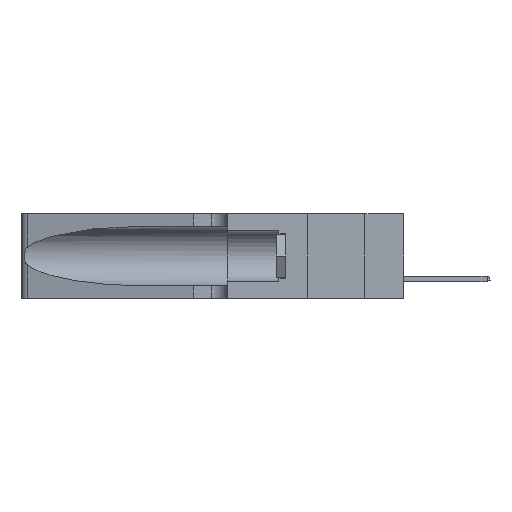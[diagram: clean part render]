
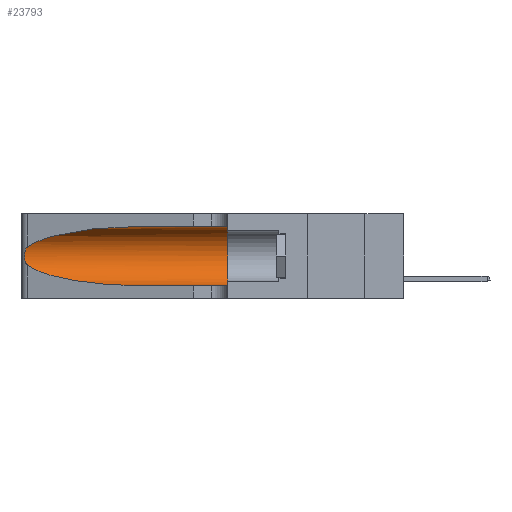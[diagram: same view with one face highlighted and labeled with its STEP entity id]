
A CAD part, left-side view. The second image highlights one B-rep face of the part: STEP entity #23793.
In plain terms, the highlighted cylindrical face has radius 3.308 mm (diameter 6.617 mm), a partial arc.
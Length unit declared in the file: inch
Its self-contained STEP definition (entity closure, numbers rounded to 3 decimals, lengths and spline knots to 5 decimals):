
#1531 = DIRECTION ( 'NONE',  ( 0., -1., 0. ) ) ;
#1923 = CARTESIAN_POINT ( 'NONE',  ( 0.26075, 1.23896, 0.19203 ) ) ;
#2465 = CARTESIAN_POINT ( 'NONE',  ( 0.2373, 1.15595, 0.28018 ) ) ;
#3826 = CARTESIAN_POINT ( 'NONE',  ( 0.1305, 1.61858, 0.31525 ) ) ;
#4246 = LINE ( 'NONE', #3826, #32758 ) ;
#4574 =( BOUNDED_CURVE ( )  B_SPLINE_CURVE ( 3, ( #13751, #26073, #12186, #14116 ),
 .UNSPECIFIED., .F., .F. ) 
 B_SPLINE_CURVE_WITH_KNOTS ( ( 4, 4 ),
 ( 3.44316, 4.71239 ),
 .UNSPECIFIED. ) 
 CURVE ( )  GEOMETRIC_REPRESENTATION_ITEM ( )  RATIONAL_B_SPLINE_CURVE ( ( 1., 0.87, 0.87, 1. ) ) 
 REPRESENTATION_ITEM ( '' )  );
#6546 = CARTESIAN_POINT ( 'NONE',  ( 0.25487, 1.22718, 0.22369 ) ) ;
#7727 = CARTESIAN_POINT ( 'NONE',  ( 0.25787, 1.23484, 0.2124 ) ) ;
#7831 = CARTESIAN_POINT ( 'NONE',  ( 0.25639, 1.23184, 0.21858 ) ) ;
#8335 = ORIENTED_EDGE ( 'NONE', *, *, #14795, .F. ) ;
#8424 = ORIENTED_EDGE ( 'NONE', *, *, #20036, .T. ) ;
#9302 = VERTEX_POINT ( 'NONE', #25267 ) ;
#9339 = CARTESIAN_POINT ( 'NONE',  ( 0.1305, 0.72297, 0.05475 ) ) ;
#10026 = CARTESIAN_POINT ( 'NONE',  ( 0.25487, 1.22718, 0.14631 ) ) ;
#10358 = CARTESIAN_POINT ( 'NONE',  ( 0.25856, 1.23593, 0.16098 ) ) ;
#10730 = CARTESIAN_POINT ( 'NONE',  ( 0.26018, 1.23835, 0.19895 ) ) ;
#10755 = DIRECTION ( 'NONE',  ( 0., 0., -1. ) ) ;
#12186 = CARTESIAN_POINT ( 'NONE',  ( 0.18966, 0.96281, 0.05475 ) ) ;
#12914 = AXIS2_PLACEMENT_3D ( 'NONE', #31276, #17505, #10755 ) ;
#12958 = DIRECTION ( 'NONE',  ( 0., -1., 0. ) ) ;
#12993 = ORIENTED_EDGE ( 'NONE', *, *, #33071, .T. ) ;
#13019 = AXIS2_PLACEMENT_3D ( 'NONE', #30638, #27631, #33396 ) ;
#13751 = CARTESIAN_POINT ( 'NONE',  ( 0.25487, 1.22718, 0.14631 ) ) ;
#13845 = B_SPLINE_CURVE_WITH_KNOTS ( 'NONE', 3,
 ( #24495, #27033, #7831, #7727, #15796, #10730, #1923, #35214, #32194, #10358, #16034, #32328, #32706, #24113 ),
 .UNSPECIFIED., .F., .F.,
 ( 4, 2, 2, 2, 2, 2, 4 ),
 ( 0., 0.00027, 0.00053, 0.00107, 0.0016, 0.00187, 0.00214 ),
 .UNSPECIFIED. ) ;
#14116 = CARTESIAN_POINT ( 'NONE',  ( 0.1305, 0.72297, 0.05475 ) ) ;
#14390 = ORIENTED_EDGE ( 'NONE', *, *, #17416, .F. ) ;
#14795 = EDGE_CURVE ( 'NONE', #35365, #9302, #4246, .T. ) ;
#15796 = CARTESIAN_POINT ( 'NONE',  ( 0.25854, 1.2359, 0.20912 ) ) ;
#16034 = CARTESIAN_POINT ( 'NONE',  ( 0.25789, 1.23486, 0.15765 ) ) ;
#16578 = VERTEX_POINT ( 'NONE', #22984 ) ;
#17416 = EDGE_CURVE ( 'NONE', #9302, #16578, #18355, .T. ) ;
#17505 = DIRECTION ( 'NONE',  ( 0., -1., 0. ) ) ;
#18355 = CIRCLE ( 'NONE', #13019, 0.13025 ) ;
#18479 = EDGE_CURVE ( 'NONE', #34839, #16578, #27793, .T. ) ;
#19209 = CARTESIAN_POINT ( 'NONE',  ( 0.25487, 1.22718, 0.22369 ) ) ;
#19756 = VERTEX_POINT ( 'NONE', #6546 ) ;
#20036 = EDGE_CURVE ( 'NONE', #32443, #34839, #4574, .T. ) ;
#20572 = EDGE_CURVE ( 'NONE', #35365, #19756, #34001, .T. ) ;
#21276 = CYLINDRICAL_SURFACE ( 'NONE', #12914, 0.13025 ) ;
#21859 = ORIENTED_EDGE ( 'NONE', *, *, #20572, .T. ) ;
#22984 = CARTESIAN_POINT ( 'NONE',  ( 0.1305, 0.35, 0.05475 ) ) ;
#23410 = FACE_OUTER_BOUND ( 'NONE', #30084, .T. ) ;
#23793 = ADVANCED_FACE ( 'NONE', ( #23410 ), #21276, .F. ) ;
#24113 = CARTESIAN_POINT ( 'NONE',  ( 0.25487, 1.22718, 0.14631 ) ) ;
#24415 = CARTESIAN_POINT ( 'NONE',  ( 0.1305, 0.72297, 0.31525 ) ) ;
#24495 = CARTESIAN_POINT ( 'NONE',  ( 0.25487, 1.22718, 0.22369 ) ) ;
#25267 = CARTESIAN_POINT ( 'NONE',  ( 0.1305, 0.35, 0.31525 ) ) ;
#25361 = CARTESIAN_POINT ( 'NONE',  ( 0.1305, 0.72297, 0.31525 ) ) ;
#26073 = CARTESIAN_POINT ( 'NONE',  ( 0.2373, 1.15595, 0.08982 ) ) ;
#27033 = CARTESIAN_POINT ( 'NONE',  ( 0.25555, 1.22994, 0.2215 ) ) ;
#27631 = DIRECTION ( 'NONE',  ( 0., 1., 0. ) ) ;
#27793 = LINE ( 'NONE', #28835, #30389 ) ;
#28835 = CARTESIAN_POINT ( 'NONE',  ( 0.1305, 1.61858, 0.05475 ) ) ;
#30084 = EDGE_LOOP ( 'NONE', ( #21859, #12993, #8424, #34900, #14390, #8335 ) ) ;
#30389 = VECTOR ( 'NONE', #12958, 39.37008 ) ;
#30638 = CARTESIAN_POINT ( 'NONE',  ( 0.1305, 0.35, 0.185 ) ) ;
#31276 = CARTESIAN_POINT ( 'NONE',  ( 0.1305, 1.61858, 0.185 ) ) ;
#32194 = CARTESIAN_POINT ( 'NONE',  ( 0.26017, 1.23833, 0.17102 ) ) ;
#32245 = CARTESIAN_POINT ( 'NONE',  ( 0.18966, 0.96281, 0.31525 ) ) ;
#32328 = CARTESIAN_POINT ( 'NONE',  ( 0.25639, 1.23186, 0.15144 ) ) ;
#32443 = VERTEX_POINT ( 'NONE', #10026 ) ;
#32706 = CARTESIAN_POINT ( 'NONE',  ( 0.25555, 1.22993, 0.14849 ) ) ;
#32758 = VECTOR ( 'NONE', #1531, 39.37008 ) ;
#33071 = EDGE_CURVE ( 'NONE', #19756, #32443, #13845, .T. ) ;
#33396 = DIRECTION ( 'NONE',  ( 0., 0., 1. ) ) ;
#34001 =( BOUNDED_CURVE ( )  B_SPLINE_CURVE ( 3, ( #24415, #32245, #2465, #19209 ),
 .UNSPECIFIED., .F., .F. ) 
 B_SPLINE_CURVE_WITH_KNOTS ( ( 4, 4 ),
 ( 1.5708, 2.84003 ),
 .UNSPECIFIED. ) 
 CURVE ( )  GEOMETRIC_REPRESENTATION_ITEM ( )  RATIONAL_B_SPLINE_CURVE ( ( 1., 0.87, 0.87, 1. ) ) 
 REPRESENTATION_ITEM ( '' )  );
#34839 = VERTEX_POINT ( 'NONE', #9339 ) ;
#34900 = ORIENTED_EDGE ( 'NONE', *, *, #18479, .T. ) ;
#35214 = CARTESIAN_POINT ( 'NONE',  ( 0.26075, 1.23896, 0.178 ) ) ;
#35365 = VERTEX_POINT ( 'NONE', #25361 ) ;
